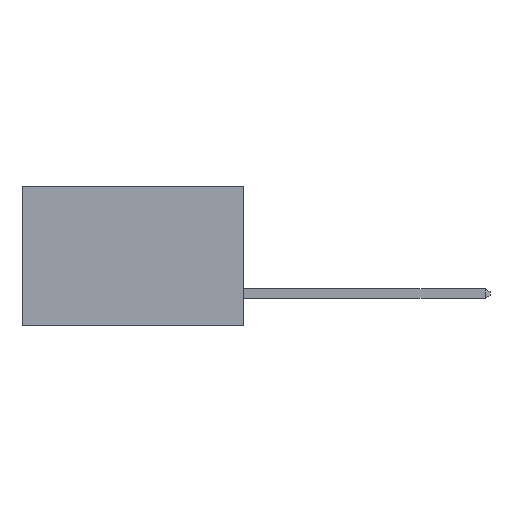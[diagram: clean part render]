
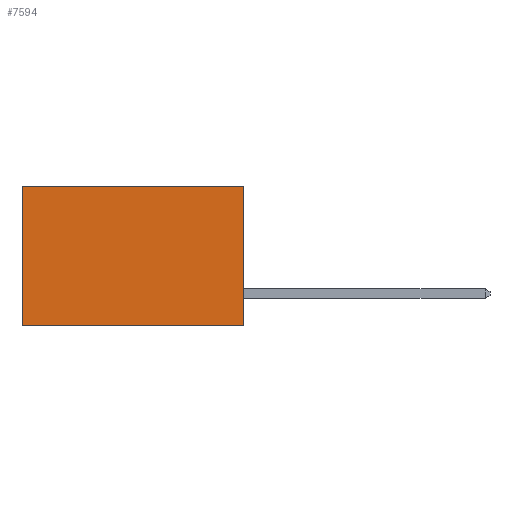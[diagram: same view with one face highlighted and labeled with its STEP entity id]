
A CAD part, left-side view. The second image highlights one B-rep face of the part: STEP entity #7594.
In plain terms, the highlighted planar face has unit normal (-1, 0, 0).
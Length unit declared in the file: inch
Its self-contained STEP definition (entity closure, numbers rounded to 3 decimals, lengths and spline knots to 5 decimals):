
#312 = CARTESIAN_POINT ( 'NONE',  ( 0.277, 0., -0.37 ) ) ;
#854 = DIRECTION ( 'NONE',  ( 0., 1., 0. ) ) ;
#869 = CARTESIAN_POINT ( 'NONE',  ( 0.277, 0.59, -0.37 ) ) ;
#1059 = CARTESIAN_POINT ( 'NONE',  ( 0.277, 0., 0. ) ) ;
#1070 = LINE ( 'NONE', #5749, #1288 ) ;
#1288 = VECTOR ( 'NONE', #5573, 39.37008 ) ;
#1576 = EDGE_LOOP ( 'NONE', ( #2029, #2217, #3032, #3212 ) ) ;
#1614 = LINE ( 'NONE', #1059, #6274 ) ;
#1755 = CARTESIAN_POINT ( 'NONE',  ( 0.277, 0.59, 0. ) ) ;
#1763 = CARTESIAN_POINT ( 'NONE',  ( 0.277, 0., 0. ) ) ;
#2029 = ORIENTED_EDGE ( 'NONE', *, *, #2703, .T. ) ;
#2080 = LINE ( 'NONE', #869, #7021 ) ;
#2217 = ORIENTED_EDGE ( 'NONE', *, *, #6408, .F. ) ;
#2222 = VERTEX_POINT ( 'NONE', #1755 ) ;
#2703 = EDGE_CURVE ( 'NONE', #2222, #7619, #2080, .T. ) ;
#2720 = FACE_OUTER_BOUND ( 'NONE', #1576, .T. ) ;
#3032 = ORIENTED_EDGE ( 'NONE', *, *, #4508, .F. ) ;
#3061 = CARTESIAN_POINT ( 'NONE',  ( 0.277, 0., -0.37 ) ) ;
#3212 = ORIENTED_EDGE ( 'NONE', *, *, #6243, .T. ) ;
#4353 = CARTESIAN_POINT ( 'NONE',  ( 0.277, 0.59, -0.37 ) ) ;
#4451 = DIRECTION ( 'NONE',  ( 0., 0., -1. ) ) ;
#4453 = DIRECTION ( 'NONE',  ( 1., 0., 0. ) ) ;
#4468 = CARTESIAN_POINT ( 'NONE',  ( 0.277, 0., -0.37 ) ) ;
#4476 = PLANE ( 'NONE',  #4551 ) ;
#4508 = EDGE_CURVE ( 'NONE', #6205, #7890, #1070, .T. ) ;
#4551 = AXIS2_PLACEMENT_3D ( 'NONE', #4468, #4453, #4451 ) ;
#5190 = VECTOR ( 'NONE', #7847, 39.37008 ) ;
#5573 = DIRECTION ( 'NONE',  ( 0., 0., -1. ) ) ;
#5749 = CARTESIAN_POINT ( 'NONE',  ( 0.277, 0., -0.37 ) ) ;
#6090 = DIRECTION ( 'NONE',  ( 0., 0., -1. ) ) ;
#6205 = VERTEX_POINT ( 'NONE', #1763 ) ;
#6243 = EDGE_CURVE ( 'NONE', #6205, #2222, #1614, .T. ) ;
#6274 = VECTOR ( 'NONE', #854, 39.37008 ) ;
#6408 = EDGE_CURVE ( 'NONE', #7890, #7619, #6726, .T. ) ;
#6726 = LINE ( 'NONE', #312, #5190 ) ;
#7021 = VECTOR ( 'NONE', #6090, 39.37008 ) ;
#7594 = ADVANCED_FACE ( 'NONE', ( #2720 ), #4476, .F. ) ;
#7619 = VERTEX_POINT ( 'NONE', #4353 ) ;
#7847 = DIRECTION ( 'NONE',  ( 0., 1., 0. ) ) ;
#7890 = VERTEX_POINT ( 'NONE', #3061 ) ;
